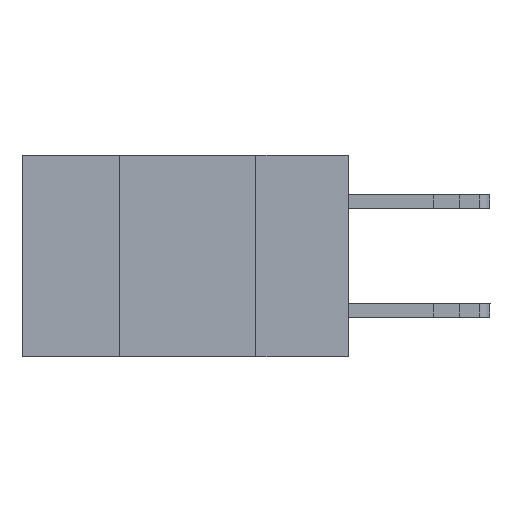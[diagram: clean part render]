
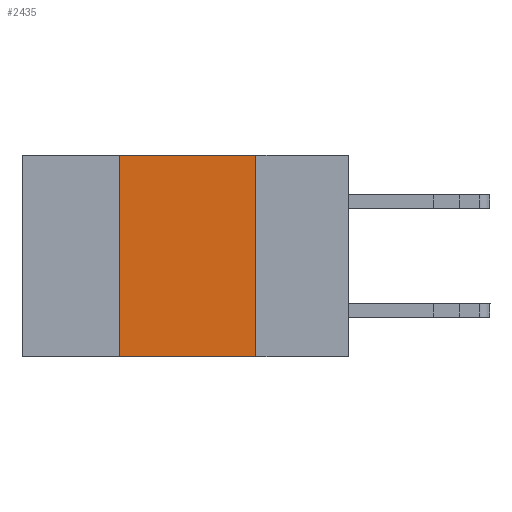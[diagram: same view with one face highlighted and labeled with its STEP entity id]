
A CAD part, left-side view. The second image highlights one B-rep face of the part: STEP entity #2435.
In plain terms, the highlighted planar face has unit normal (-1, 0, 0).
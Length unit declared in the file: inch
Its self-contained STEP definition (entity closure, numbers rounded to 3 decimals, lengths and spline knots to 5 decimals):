
#589 = VECTOR ( 'NONE', #10468, 39.37008 ) ;
#1027 = VECTOR ( 'NONE', #6316, 39.37008 ) ;
#1180 = LINE ( 'NONE', #2227, #11287 ) ;
#1203 = DIRECTION ( 'NONE',  ( 1., 0., 0. ) ) ;
#2225 = DIRECTION ( 'NONE',  ( 0., 0., -1. ) ) ;
#2227 = CARTESIAN_POINT ( 'NONE',  ( 0., 0.17, -0.37 ) ) ;
#2305 = LINE ( 'NONE', #7737, #6557 ) ;
#2435 = ADVANCED_FACE ( 'NONE', ( #12278 ), #5654, .F. ) ;
#2523 = CARTESIAN_POINT ( 'NONE',  ( 0., 0.17, 0. ) ) ;
#2566 = VERTEX_POINT ( 'NONE', #9708 ) ;
#2608 = EDGE_CURVE ( 'NONE', #8238, #4715, #2305, .T. ) ;
#2971 = EDGE_CURVE ( 'NONE', #8238, #2566, #4058, .T. ) ;
#3669 = LINE ( 'NONE', #9599, #589 ) ;
#3836 = EDGE_CURVE ( 'NONE', #9612, #4715, #1180, .T. ) ;
#4058 = LINE ( 'NONE', #7677, #1027 ) ;
#4715 = VERTEX_POINT ( 'NONE', #9313 ) ;
#5011 = DIRECTION ( 'NONE',  ( 0., 0., -1. ) ) ;
#5516 = ORIENTED_EDGE ( 'NONE', *, *, #2971, .F. ) ;
#5654 = PLANE ( 'NONE',  #10569 ) ;
#5812 = EDGE_CURVE ( 'NONE', #2566, #9612, #3669, .T. ) ;
#6312 = CARTESIAN_POINT ( 'NONE',  ( 0., 0.6, 0. ) ) ;
#6316 = DIRECTION ( 'NONE',  ( 0., 0., 1. ) ) ;
#6557 = VECTOR ( 'NONE', #7477, 39.37008 ) ;
#7477 = DIRECTION ( 'NONE',  ( 0., -1., 0. ) ) ;
#7677 = CARTESIAN_POINT ( 'NONE',  ( 0., 0.42, -0.37 ) ) ;
#7682 = ORIENTED_EDGE ( 'NONE', *, *, #3836, .F. ) ;
#7737 = CARTESIAN_POINT ( 'NONE',  ( 0., 0.6, -0.37 ) ) ;
#7959 = ORIENTED_EDGE ( 'NONE', *, *, #2608, .T. ) ;
#8238 = VERTEX_POINT ( 'NONE', #11595 ) ;
#8394 = EDGE_LOOP ( 'NONE', ( #7682, #10064, #5516, #7959 ) ) ;
#9313 = CARTESIAN_POINT ( 'NONE',  ( 0., 0.17, -0.37 ) ) ;
#9599 = CARTESIAN_POINT ( 'NONE',  ( 0., 0.6, 0. ) ) ;
#9612 = VERTEX_POINT ( 'NONE', #2523 ) ;
#9708 = CARTESIAN_POINT ( 'NONE',  ( 0., 0.42, 0. ) ) ;
#10064 = ORIENTED_EDGE ( 'NONE', *, *, #5812, .F. ) ;
#10468 = DIRECTION ( 'NONE',  ( 0., -1., 0. ) ) ;
#10569 = AXIS2_PLACEMENT_3D ( 'NONE', #6312, #1203, #5011 ) ;
#11287 = VECTOR ( 'NONE', #2225, 39.37008 ) ;
#11595 = CARTESIAN_POINT ( 'NONE',  ( 0., 0.42, -0.37 ) ) ;
#12278 = FACE_OUTER_BOUND ( 'NONE', #8394, .T. ) ;
